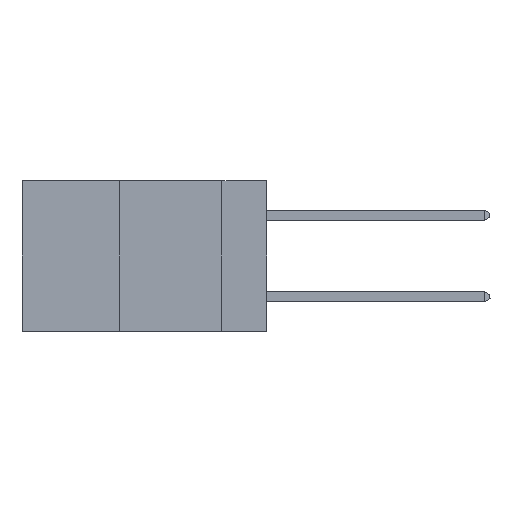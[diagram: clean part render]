
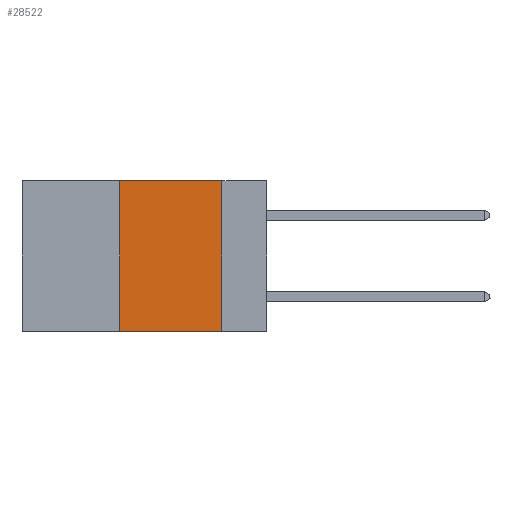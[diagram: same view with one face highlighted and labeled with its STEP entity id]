
A CAD part, left-side view. The second image highlights one B-rep face of the part: STEP entity #28522.
In plain terms, the highlighted planar face has unit normal (-1, 0, 0).
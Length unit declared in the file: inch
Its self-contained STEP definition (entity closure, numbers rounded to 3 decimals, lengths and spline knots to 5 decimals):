
#562 = ORIENTED_EDGE ( 'NONE', *, *, #6055, .F. ) ;
#1078 = CARTESIAN_POINT ( 'NONE',  ( 0., 0.6, 0. ) ) ;
#1542 = CARTESIAN_POINT ( 'NONE',  ( 0., 0.36, 0. ) ) ;
#1805 = CARTESIAN_POINT ( 'NONE',  ( 0., 0.36, 0. ) ) ;
#1867 = VECTOR ( 'NONE', #27627, 39.37008 ) ;
#2063 = VECTOR ( 'NONE', #24211, 39.37008 ) ;
#2953 = CARTESIAN_POINT ( 'NONE',  ( 0., 0.11, 0. ) ) ;
#3946 = PLANE ( 'NONE',  #12683 ) ;
#4402 = ORIENTED_EDGE ( 'NONE', *, *, #7281, .F. ) ;
#4613 = EDGE_CURVE ( 'NONE', #18201, #23712, #5358, .T. ) ;
#5078 = CARTESIAN_POINT ( 'NONE',  ( 0., 0.6, -0.37 ) ) ;
#5358 = LINE ( 'NONE', #5078, #1867 ) ;
#6055 = EDGE_CURVE ( 'NONE', #26992, #23712, #22529, .T. ) ;
#7281 = EDGE_CURVE ( 'NONE', #24601, #26992, #10708, .T. ) ;
#7812 = EDGE_CURVE ( 'NONE', #18201, #24601, #11811, .T. ) ;
#8021 = DIRECTION ( 'NONE',  ( 0., 0., -1. ) ) ;
#10439 = ORIENTED_EDGE ( 'NONE', *, *, #7812, .F. ) ;
#10605 = EDGE_LOOP ( 'NONE', ( #562, #4402, #10439, #23449 ) ) ;
#10708 = LINE ( 'NONE', #1078, #21257 ) ;
#11811 = LINE ( 'NONE', #1805, #2063 ) ;
#12396 = CARTESIAN_POINT ( 'NONE',  ( 0., 0.36, -0.37 ) ) ;
#12683 = AXIS2_PLACEMENT_3D ( 'NONE', #28667, #23748, #13860 ) ;
#13860 = DIRECTION ( 'NONE',  ( 0., 0., -1. ) ) ;
#15872 = VECTOR ( 'NONE', #8021, 39.37008 ) ;
#18201 = VERTEX_POINT ( 'NONE', #12396 ) ;
#20697 = CARTESIAN_POINT ( 'NONE',  ( 0., 0.11, 0. ) ) ;
#21257 = VECTOR ( 'NONE', #30930, 39.37008 ) ;
#22529 = LINE ( 'NONE', #20697, #15872 ) ;
#23449 = ORIENTED_EDGE ( 'NONE', *, *, #4613, .T. ) ;
#23712 = VERTEX_POINT ( 'NONE', #27388 ) ;
#23748 = DIRECTION ( 'NONE',  ( 1., 0., 0. ) ) ;
#24211 = DIRECTION ( 'NONE',  ( 0., 0., 1. ) ) ;
#24601 = VERTEX_POINT ( 'NONE', #1542 ) ;
#26768 = FACE_OUTER_BOUND ( 'NONE', #10605, .T. ) ;
#26992 = VERTEX_POINT ( 'NONE', #2953 ) ;
#27388 = CARTESIAN_POINT ( 'NONE',  ( 0., 0.11, -0.37 ) ) ;
#27627 = DIRECTION ( 'NONE',  ( 0., -1., 0. ) ) ;
#28522 = ADVANCED_FACE ( 'NONE', ( #26768 ), #3946, .F. ) ;
#28667 = CARTESIAN_POINT ( 'NONE',  ( 0., 0.6, 0. ) ) ;
#30930 = DIRECTION ( 'NONE',  ( 0., -1., 0. ) ) ;
